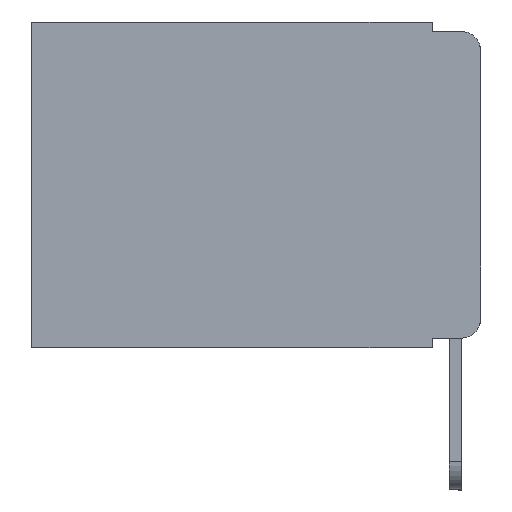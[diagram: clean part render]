
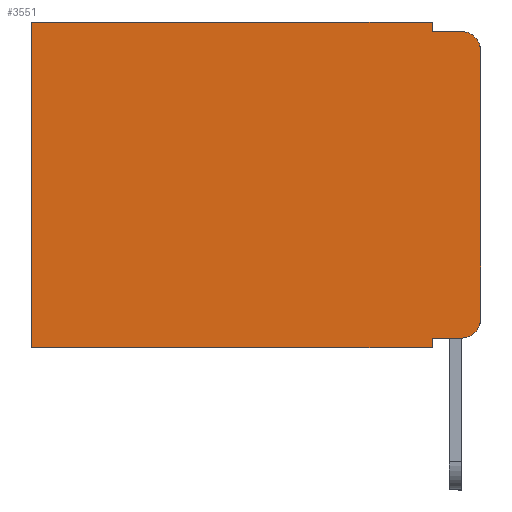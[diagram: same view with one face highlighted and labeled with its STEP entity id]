
A CAD part, left-side view. The second image highlights one B-rep face of the part: STEP entity #3551.
In plain terms, the highlighted planar face has unit normal (-1, 0, 0).
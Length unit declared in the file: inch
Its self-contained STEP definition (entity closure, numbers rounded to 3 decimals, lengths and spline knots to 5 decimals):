
#186 = EDGE_CURVE ( 'NONE', #8100, #575, #19960, .T. ) ;
#575 = VERTEX_POINT ( 'NONE', #17972 ) ;
#758 = CARTESIAN_POINT ( 'NONE',  ( 0.298, 0.473, -0.343 ) ) ;
#839 = EDGE_CURVE ( 'NONE', #575, #1842, #6745, .T. ) ;
#902 = EDGE_CURVE ( 'NONE', #1519, #13966, #8671, .T. ) ;
#1099 = VECTOR ( 'NONE', #4839, 39.37008 ) ;
#1412 = ORIENTED_EDGE ( 'NONE', *, *, #16775, .T. ) ;
#1519 = VERTEX_POINT ( 'NONE', #14989 ) ;
#1552 = EDGE_CURVE ( 'NONE', #16777, #17105, #15206, .T. ) ;
#1842 = VERTEX_POINT ( 'NONE', #14227 ) ;
#1926 = VERTEX_POINT ( 'NONE', #14775 ) ;
#2948 = CARTESIAN_POINT ( 'NONE',  ( 0.298, 0., -0.313 ) ) ;
#2988 = ORIENTED_EDGE ( 'NONE', *, *, #902, .F. ) ;
#3551 = ADVANCED_FACE ( 'NONE', ( #10965 ), #15843, .F. ) ;
#3760 = VERTEX_POINT ( 'NONE', #13042 ) ;
#4177 = LINE ( 'NONE', #4394, #11752 ) ;
#4203 = VECTOR ( 'NONE', #18901, 39.37008 ) ;
#4394 = CARTESIAN_POINT ( 'NONE',  ( 0.298, 0.051, -0.333 ) ) ;
#4466 = CIRCLE ( 'NONE', #7332, 0.02 ) ;
#4573 = EDGE_CURVE ( 'NONE', #3760, #1926, #4177, .T. ) ;
#4654 = EDGE_CURVE ( 'NONE', #16138, #17105, #11636, .T. ) ;
#4839 = DIRECTION ( 'NONE',  ( 0., 0., -1. ) ) ;
#5479 = CARTESIAN_POINT ( 'NONE',  ( 0.298, 0.473, 0. ) ) ;
#5821 = DIRECTION ( 'NONE',  ( 1., 0., 0. ) ) ;
#5886 = ORIENTED_EDGE ( 'NONE', *, *, #10882, .T. ) ;
#6181 = DIRECTION ( 'NONE',  ( 0., 0., -1. ) ) ;
#6392 = CARTESIAN_POINT ( 'NONE',  ( 0.298, 0.051, 0. ) ) ;
#6745 = LINE ( 'NONE', #6793, #11684 ) ;
#6793 = CARTESIAN_POINT ( 'NONE',  ( 0.298, 0.051, -0.01 ) ) ;
#7190 = DIRECTION ( 'NONE',  ( 0., 1., 0. ) ) ;
#7332 = AXIS2_PLACEMENT_3D ( 'NONE', #14664, #8204, #21690 ) ;
#7865 = ORIENTED_EDGE ( 'NONE', *, *, #4573, .T. ) ;
#8100 = VERTEX_POINT ( 'NONE', #15801 ) ;
#8106 = ORIENTED_EDGE ( 'NONE', *, *, #1552, .F. ) ;
#8204 = DIRECTION ( 'NONE',  ( -1., 0., 0. ) ) ;
#8671 = LINE ( 'NONE', #15442, #4203 ) ;
#9259 = LINE ( 'NONE', #16132, #17928 ) ;
#9288 = DIRECTION ( 'NONE',  ( 0., 0., -1. ) ) ;
#9461 = AXIS2_PLACEMENT_3D ( 'NONE', #15868, #11193, #6181 ) ;
#10669 = AXIS2_PLACEMENT_3D ( 'NONE', #19522, #5821, #9288 ) ;
#10882 = EDGE_CURVE ( 'NONE', #1926, #13966, #4466, .T. ) ;
#10899 = ORIENTED_EDGE ( 'NONE', *, *, #839, .F. ) ;
#10965 = FACE_OUTER_BOUND ( 'NONE', #19584, .T. ) ;
#11193 = DIRECTION ( 'NONE',  ( -1., 0., 0. ) ) ;
#11481 = VECTOR ( 'NONE', #21421, 39.37008 ) ;
#11561 = ORIENTED_EDGE ( 'NONE', *, *, #4654, .T. ) ;
#11636 = LINE ( 'NONE', #16851, #1099 ) ;
#11645 = VECTOR ( 'NONE', #7190, 39.37008 ) ;
#11684 = VECTOR ( 'NONE', #17121, 39.37008 ) ;
#11752 = VECTOR ( 'NONE', #12965, 39.37008 ) ;
#12965 = DIRECTION ( 'NONE',  ( 0., -1., 0. ) ) ;
#13042 = CARTESIAN_POINT ( 'NONE',  ( 0.298, 0.051, -0.333 ) ) ;
#13053 = LINE ( 'NONE', #19745, #11481 ) ;
#13966 = VERTEX_POINT ( 'NONE', #2948 ) ;
#14192 = CARTESIAN_POINT ( 'NONE',  ( 0.298, 0., -0.343 ) ) ;
#14227 = CARTESIAN_POINT ( 'NONE',  ( 0.298, 0.02, -0.01 ) ) ;
#14664 = CARTESIAN_POINT ( 'NONE',  ( 0.298, 0.02, -0.313 ) ) ;
#14665 = EDGE_CURVE ( 'NONE', #3760, #16777, #13053, .T. ) ;
#14775 = CARTESIAN_POINT ( 'NONE',  ( 0.298, 0.02, -0.333 ) ) ;
#14989 = CARTESIAN_POINT ( 'NONE',  ( 0.298, 0., -0.03 ) ) ;
#15206 = LINE ( 'NONE', #14192, #11645 ) ;
#15442 = CARTESIAN_POINT ( 'NONE',  ( 0.298, 0., 0. ) ) ;
#15801 = CARTESIAN_POINT ( 'NONE',  ( 0.298, 0.051, 0. ) ) ;
#15843 = PLANE ( 'NONE',  #10669 ) ;
#15868 = CARTESIAN_POINT ( 'NONE',  ( 0.298, 0.02, -0.03 ) ) ;
#16033 = CARTESIAN_POINT ( 'NONE',  ( 0.298, 0.051, -0.343 ) ) ;
#16132 = CARTESIAN_POINT ( 'NONE',  ( 0.298, 0., 0. ) ) ;
#16138 = VERTEX_POINT ( 'NONE', #5479 ) ;
#16244 = DIRECTION ( 'NONE',  ( 0., 1., 0. ) ) ;
#16605 = ORIENTED_EDGE ( 'NONE', *, *, #17621, .T. ) ;
#16775 = EDGE_CURVE ( 'NONE', #8100, #16138, #9259, .T. ) ;
#16777 = VERTEX_POINT ( 'NONE', #16033 ) ;
#16851 = CARTESIAN_POINT ( 'NONE',  ( 0.298, 0.473, 0. ) ) ;
#17105 = VERTEX_POINT ( 'NONE', #758 ) ;
#17121 = DIRECTION ( 'NONE',  ( 0., -1., 0. ) ) ;
#17621 = EDGE_CURVE ( 'NONE', #1519, #1842, #19032, .T. ) ;
#17928 = VECTOR ( 'NONE', #16244, 39.37008 ) ;
#17972 = CARTESIAN_POINT ( 'NONE',  ( 0.298, 0.051, -0.01 ) ) ;
#18901 = DIRECTION ( 'NONE',  ( 0., 0., -1. ) ) ;
#19032 = CIRCLE ( 'NONE', #9461, 0.02 ) ;
#19329 = ORIENTED_EDGE ( 'NONE', *, *, #186, .F. ) ;
#19522 = CARTESIAN_POINT ( 'NONE',  ( 0.298, 0., 0. ) ) ;
#19584 = EDGE_LOOP ( 'NONE', ( #2988, #16605, #10899, #19329, #1412, #11561, #8106, #21693, #7865, #5886 ) ) ;
#19745 = CARTESIAN_POINT ( 'NONE',  ( 0.298, 0.051, 0. ) ) ;
#19960 = LINE ( 'NONE', #6392, #21172 ) ;
#21172 = VECTOR ( 'NONE', #21975, 39.37008 ) ;
#21421 = DIRECTION ( 'NONE',  ( 0., 0., -1. ) ) ;
#21690 = DIRECTION ( 'NONE',  ( 0., 0., -1. ) ) ;
#21693 = ORIENTED_EDGE ( 'NONE', *, *, #14665, .F. ) ;
#21975 = DIRECTION ( 'NONE',  ( 0., 0., -1. ) ) ;
